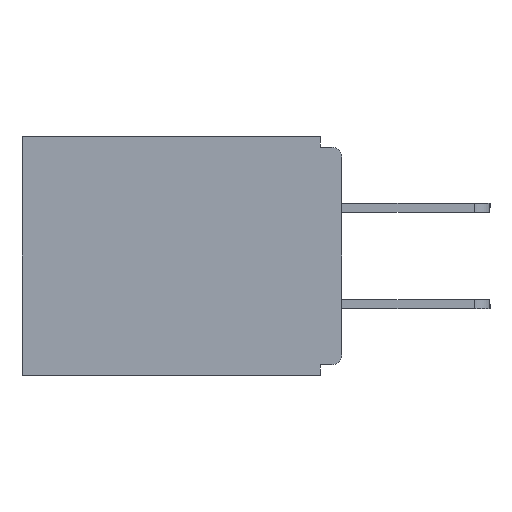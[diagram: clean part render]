
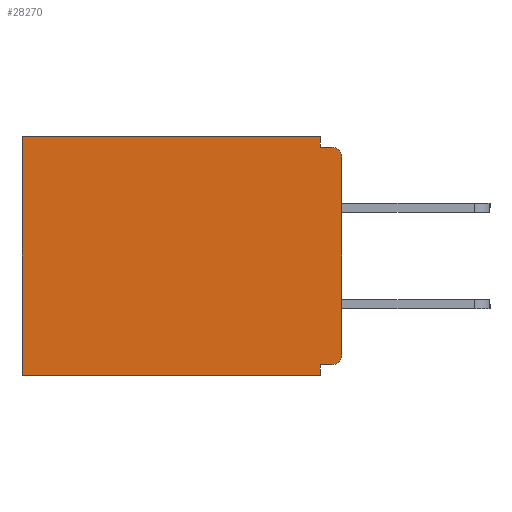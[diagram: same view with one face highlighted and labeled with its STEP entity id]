
A CAD part, left-side view. The second image highlights one B-rep face of the part: STEP entity #28270.
In plain terms, the highlighted planar face has unit normal (-1, 0, 0).
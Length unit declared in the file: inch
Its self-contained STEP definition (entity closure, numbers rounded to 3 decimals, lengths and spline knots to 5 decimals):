
#425 = VERTEX_POINT ( 'NONE', #10505 ) ;
#670 = DIRECTION ( 'NONE',  ( -1., 0., 0. ) ) ;
#1798 = VECTOR ( 'NONE', #5599, 39.37008 ) ;
#2532 = LINE ( 'NONE', #29448, #1798 ) ;
#2804 = DIRECTION ( 'NONE',  ( -1., 0., 0. ) ) ;
#2841 = CARTESIAN_POINT ( 'NONE',  ( 0.298, 0., -0.313 ) ) ;
#3416 = AXIS2_PLACEMENT_3D ( 'NONE', #14865, #670, #17240 ) ;
#3601 = VECTOR ( 'NONE', #8711, 39.37008 ) ;
#4417 = AXIS2_PLACEMENT_3D ( 'NONE', #21859, #2804, #5167 ) ;
#4558 = CARTESIAN_POINT ( 'NONE',  ( 0.298, 0., -0.03 ) ) ;
#5167 = DIRECTION ( 'NONE',  ( 0., 0., -1. ) ) ;
#5599 = DIRECTION ( 'NONE',  ( 0., -1., 0. ) ) ;
#6045 = VERTEX_POINT ( 'NONE', #21456 ) ;
#6262 = EDGE_CURVE ( 'NONE', #29556, #15161, #29502, .T. ) ;
#6563 = ORIENTED_EDGE ( 'NONE', *, *, #24192, .F. ) ;
#7308 = LINE ( 'NONE', #30259, #3601 ) ;
#7589 = VECTOR ( 'NONE', #27756, 39.37008 ) ;
#7925 = EDGE_CURVE ( 'NONE', #6045, #23290, #21567, .T. ) ;
#8711 = DIRECTION ( 'NONE',  ( 0., 0., -1. ) ) ;
#9288 = ORIENTED_EDGE ( 'NONE', *, *, #18069, .F. ) ;
#10178 = DIRECTION ( 'NONE',  ( 0., 1., 0. ) ) ;
#10505 = CARTESIAN_POINT ( 'NONE',  ( 0.298, 0.031, -0.015 ) ) ;
#10512 = ORIENTED_EDGE ( 'NONE', *, *, #12203, .T. ) ;
#10626 = CARTESIAN_POINT ( 'NONE',  ( 0.298, 0.031, -0.343 ) ) ;
#10645 = DIRECTION ( 'NONE',  ( 0., 1., 0. ) ) ;
#10694 = ORIENTED_EDGE ( 'NONE', *, *, #18093, .F. ) ;
#11190 = VECTOR ( 'NONE', #10645, 39.37008 ) ;
#11264 = EDGE_CURVE ( 'NONE', #30422, #18882, #7308, .T. ) ;
#11269 = EDGE_LOOP ( 'NONE', ( #14631, #10694, #23767, #14608, #26883, #6563, #28574, #9288, #10512, #17550 ) ) ;
#12203 = EDGE_CURVE ( 'NONE', #25270, #18882, #20521, .T. ) ;
#12206 = CARTESIAN_POINT ( 'NONE',  ( 0.298, 0.015, -0.328 ) ) ;
#12968 = CARTESIAN_POINT ( 'NONE',  ( 0.298, 0., -0.343 ) ) ;
#13943 = LINE ( 'NONE', #20567, #7589 ) ;
#14517 = LINE ( 'NONE', #10626, #28985 ) ;
#14608 = ORIENTED_EDGE ( 'NONE', *, *, #17656, .T. ) ;
#14631 = ORIENTED_EDGE ( 'NONE', *, *, #22491, .T. ) ;
#14658 = VECTOR ( 'NONE', #17900, 39.37008 ) ;
#14865 = CARTESIAN_POINT ( 'NONE',  ( 0.298, 0.015, -0.313 ) ) ;
#14979 = CARTESIAN_POINT ( 'NONE',  ( 0.298, 0.031, 0. ) ) ;
#15161 = VERTEX_POINT ( 'NONE', #28498 ) ;
#15198 = DIRECTION ( 'NONE',  ( 1., 0., 0. ) ) ;
#15393 = DIRECTION ( 'NONE',  ( 0., 0., -1. ) ) ;
#16415 = CARTESIAN_POINT ( 'NONE',  ( 0.298, 0.031, -0.343 ) ) ;
#17055 = VERTEX_POINT ( 'NONE', #14979 ) ;
#17240 = DIRECTION ( 'NONE',  ( 0., 0., -1. ) ) ;
#17550 = ORIENTED_EDGE ( 'NONE', *, *, #11264, .F. ) ;
#17656 = EDGE_CURVE ( 'NONE', #17055, #29556, #13943, .T. ) ;
#17772 = PLANE ( 'NONE',  #22345 ) ;
#17900 = DIRECTION ( 'NONE',  ( 0., 0., -1. ) ) ;
#18069 = EDGE_CURVE ( 'NONE', #25270, #6045, #28532, .T. ) ;
#18093 = EDGE_CURVE ( 'NONE', #425, #22399, #2532, .T. ) ;
#18882 = VERTEX_POINT ( 'NONE', #2841 ) ;
#19212 = CARTESIAN_POINT ( 'NONE',  ( 0.298, 0.46, 0. ) ) ;
#19685 = CARTESIAN_POINT ( 'NONE',  ( 0.298, 0., -0.328 ) ) ;
#20149 = CARTESIAN_POINT ( 'NONE',  ( 0.298, 0., 0. ) ) ;
#20168 = CARTESIAN_POINT ( 'NONE',  ( 0.298, 0.46, 0. ) ) ;
#20521 = CIRCLE ( 'NONE', #3416, 0.015 ) ;
#20567 = CARTESIAN_POINT ( 'NONE',  ( 0.298, 0., 0. ) ) ;
#21456 = CARTESIAN_POINT ( 'NONE',  ( 0.298, 0.031, -0.328 ) ) ;
#21567 = LINE ( 'NONE', #16415, #27165 ) ;
#21859 = CARTESIAN_POINT ( 'NONE',  ( 0.298, 0.015, -0.03 ) ) ;
#22189 = VECTOR ( 'NONE', #10178, 39.37008 ) ;
#22225 = FACE_OUTER_BOUND ( 'NONE', #11269, .T. ) ;
#22323 = DIRECTION ( 'NONE',  ( 0., 0., -1. ) ) ;
#22345 = AXIS2_PLACEMENT_3D ( 'NONE', #20149, #15198, #22323 ) ;
#22399 = VERTEX_POINT ( 'NONE', #30567 ) ;
#22491 = EDGE_CURVE ( 'NONE', #30422, #22399, #23119, .T. ) ;
#23005 = CARTESIAN_POINT ( 'NONE',  ( 0.298, 0.031, -0.343 ) ) ;
#23119 = CIRCLE ( 'NONE', #4417, 0.015 ) ;
#23290 = VERTEX_POINT ( 'NONE', #23005 ) ;
#23767 = ORIENTED_EDGE ( 'NONE', *, *, #27556, .F. ) ;
#24192 = EDGE_CURVE ( 'NONE', #23290, #15161, #24530, .T. ) ;
#24530 = LINE ( 'NONE', #12968, #11190 ) ;
#25270 = VERTEX_POINT ( 'NONE', #12206 ) ;
#26754 = DIRECTION ( 'NONE',  ( 0., 0., -1. ) ) ;
#26883 = ORIENTED_EDGE ( 'NONE', *, *, #6262, .T. ) ;
#27165 = VECTOR ( 'NONE', #26754, 39.37008 ) ;
#27556 = EDGE_CURVE ( 'NONE', #17055, #425, #14517, .T. ) ;
#27756 = DIRECTION ( 'NONE',  ( 0., 1., 0. ) ) ;
#28270 = ADVANCED_FACE ( 'NONE', ( #22225 ), #17772, .F. ) ;
#28498 = CARTESIAN_POINT ( 'NONE',  ( 0.298, 0.46, -0.343 ) ) ;
#28532 = LINE ( 'NONE', #19685, #22189 ) ;
#28574 = ORIENTED_EDGE ( 'NONE', *, *, #7925, .F. ) ;
#28985 = VECTOR ( 'NONE', #15393, 39.37008 ) ;
#29448 = CARTESIAN_POINT ( 'NONE',  ( 0.298, 0., -0.015 ) ) ;
#29502 = LINE ( 'NONE', #20168, #14658 ) ;
#29556 = VERTEX_POINT ( 'NONE', #19212 ) ;
#30259 = CARTESIAN_POINT ( 'NONE',  ( 0.298, 0., 0. ) ) ;
#30422 = VERTEX_POINT ( 'NONE', #4558 ) ;
#30567 = CARTESIAN_POINT ( 'NONE',  ( 0.298, 0.015, -0.015 ) ) ;
